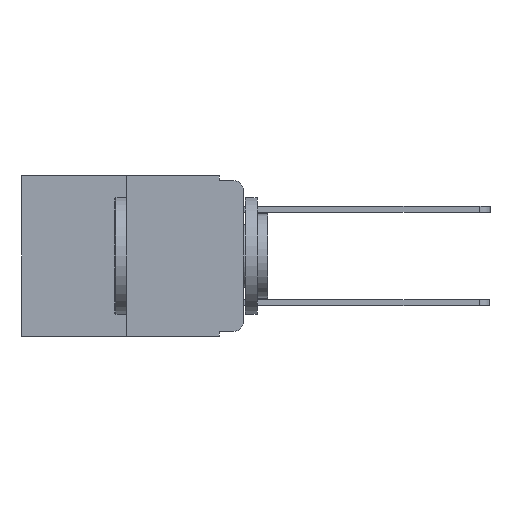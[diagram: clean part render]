
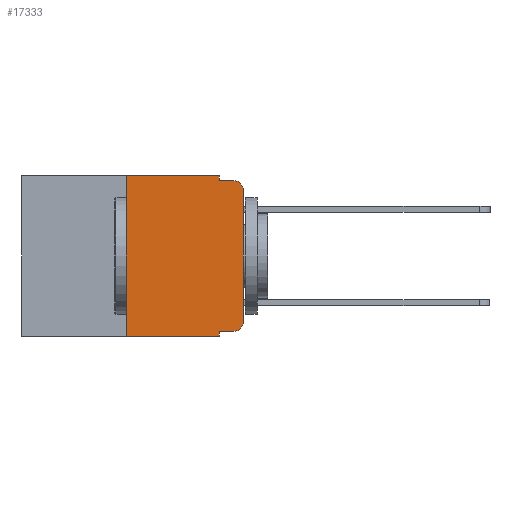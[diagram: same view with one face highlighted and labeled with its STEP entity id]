
A CAD part, left-side view. The second image highlights one B-rep face of the part: STEP entity #17333.
In plain terms, the highlighted planar face has unit normal (-1, 0, 0).
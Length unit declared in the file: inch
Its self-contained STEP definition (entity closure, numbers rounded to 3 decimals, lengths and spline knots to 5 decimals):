
#439 = CARTESIAN_POINT ( 'NONE',  ( 0., 0., -0.313 ) ) ;
#488 = CARTESIAN_POINT ( 'NONE',  ( 0., 0., 0. ) ) ;
#549 = VECTOR ( 'NONE', #4475, 39.37008 ) ;
#576 = CARTESIAN_POINT ( 'NONE',  ( 0., 0.473, 0. ) ) ;
#746 = DIRECTION ( 'NONE',  ( 0., 0., -1. ) ) ;
#815 = VERTEX_POINT ( 'NONE', #5910 ) ;
#910 = CARTESIAN_POINT ( 'NONE',  ( 0., 0.25, 0. ) ) ;
#1171 = LINE ( 'NONE', #17532, #549 ) ;
#1266 = VERTEX_POINT ( 'NONE', #5504 ) ;
#1741 = CIRCLE ( 'NONE', #10800, 0.02 ) ;
#1796 = VERTEX_POINT ( 'NONE', #20840 ) ;
#1843 = VERTEX_POINT ( 'NONE', #439 ) ;
#2025 = AXIS2_PLACEMENT_3D ( 'NONE', #576, #13933, #2569 ) ;
#2287 = CARTESIAN_POINT ( 'NONE',  ( 0., 0.051, -0.343 ) ) ;
#2481 = DIRECTION ( 'NONE',  ( 0., 0., 1. ) ) ;
#2569 = DIRECTION ( 'NONE',  ( 0., 0., -1. ) ) ;
#2634 = ORIENTED_EDGE ( 'NONE', *, *, #16061, .T. ) ;
#2987 = LINE ( 'NONE', #488, #16797 ) ;
#3080 = ORIENTED_EDGE ( 'NONE', *, *, #11273, .T. ) ;
#3301 = ORIENTED_EDGE ( 'NONE', *, *, #13153, .F. ) ;
#3503 = EDGE_CURVE ( 'NONE', #17056, #20672, #16402, .T. ) ;
#3620 = CARTESIAN_POINT ( 'NONE',  ( 0., 0.02, -0.01 ) ) ;
#3625 = ORIENTED_EDGE ( 'NONE', *, *, #6654, .T. ) ;
#3808 = ORIENTED_EDGE ( 'NONE', *, *, #7191, .F. ) ;
#3972 = EDGE_LOOP ( 'NONE', ( #4628, #7762, #17197, #21349, #4101, #3808, #3625, #3301, #3080, #2634 ) ) ;
#4101 = ORIENTED_EDGE ( 'NONE', *, *, #13943, .F. ) ;
#4105 = CARTESIAN_POINT ( 'NONE',  ( 0., 0.473, -0.343 ) ) ;
#4463 = VERTEX_POINT ( 'NONE', #2287 ) ;
#4475 = DIRECTION ( 'NONE',  ( 0., -1., 0. ) ) ;
#4520 = CARTESIAN_POINT ( 'NONE',  ( 0., 0.02, -0.313 ) ) ;
#4608 = LINE ( 'NONE', #11537, #22492 ) ;
#4628 = ORIENTED_EDGE ( 'NONE', *, *, #20937, .T. ) ;
#5504 = CARTESIAN_POINT ( 'NONE',  ( 0., 0.051, 0. ) ) ;
#5910 = CARTESIAN_POINT ( 'NONE',  ( 0., 0.25, -0.343 ) ) ;
#6438 = DIRECTION ( 'NONE',  ( 0., 0., -1. ) ) ;
#6467 = VECTOR ( 'NONE', #9586, 39.37008 ) ;
#6654 = EDGE_CURVE ( 'NONE', #815, #4463, #15599, .T. ) ;
#6898 = VERTEX_POINT ( 'NONE', #910 ) ;
#7191 = EDGE_CURVE ( 'NONE', #815, #6898, #23216, .T. ) ;
#7267 = CARTESIAN_POINT ( 'NONE',  ( 0., 0.02, -0.333 ) ) ;
#7762 = ORIENTED_EDGE ( 'NONE', *, *, #11163, .T. ) ;
#8779 = CARTESIAN_POINT ( 'NONE',  ( 0., 0.051, -0.333 ) ) ;
#8798 = CARTESIAN_POINT ( 'NONE',  ( 0., 0.051, 0. ) ) ;
#8963 = CIRCLE ( 'NONE', #15830, 0.02 ) ;
#9578 = LINE ( 'NONE', #8779, #13952 ) ;
#9586 = DIRECTION ( 'NONE',  ( 0., -1., 0. ) ) ;
#10800 = AXIS2_PLACEMENT_3D ( 'NONE', #23080, #12233, #746 ) ;
#11163 = EDGE_CURVE ( 'NONE', #1796, #20672, #1741, .T. ) ;
#11273 = EDGE_CURVE ( 'NONE', #15095, #22712, #9578, .T. ) ;
#11386 = CARTESIAN_POINT ( 'NONE',  ( 0., 0.25, 0. ) ) ;
#11537 = CARTESIAN_POINT ( 'NONE',  ( 0., 0.051, 0. ) ) ;
#12068 = PLANE ( 'NONE',  #2025 ) ;
#12233 = DIRECTION ( 'NONE',  ( -1., 0., 0. ) ) ;
#13153 = EDGE_CURVE ( 'NONE', #15095, #4463, #4608, .T. ) ;
#13527 = DIRECTION ( 'NONE',  ( 0., -1., 0. ) ) ;
#13933 = DIRECTION ( 'NONE',  ( 1., 0., 0. ) ) ;
#13943 = EDGE_CURVE ( 'NONE', #6898, #1266, #1171, .T. ) ;
#13952 = VECTOR ( 'NONE', #19811, 39.37008 ) ;
#14111 = EDGE_CURVE ( 'NONE', #1266, #17056, #21904, .T. ) ;
#14778 = CARTESIAN_POINT ( 'NONE',  ( 0., 0.051, -0.01 ) ) ;
#15026 = VECTOR ( 'NONE', #13527, 39.37008 ) ;
#15095 = VERTEX_POINT ( 'NONE', #22817 ) ;
#15599 = LINE ( 'NONE', #4105, #15026 ) ;
#15830 = AXIS2_PLACEMENT_3D ( 'NONE', #4520, #17580, #6438 ) ;
#16004 = VECTOR ( 'NONE', #23408, 39.37008 ) ;
#16061 = EDGE_CURVE ( 'NONE', #22712, #1843, #8963, .T. ) ;
#16402 = LINE ( 'NONE', #14778, #6467 ) ;
#16797 = VECTOR ( 'NONE', #2481, 39.37008 ) ;
#17056 = VERTEX_POINT ( 'NONE', #23959 ) ;
#17197 = ORIENTED_EDGE ( 'NONE', *, *, #3503, .F. ) ;
#17333 = ADVANCED_FACE ( 'NONE', ( #18134 ), #12068, .F. ) ;
#17532 = CARTESIAN_POINT ( 'NONE',  ( 0., 0.473, 0. ) ) ;
#17580 = DIRECTION ( 'NONE',  ( -1., 0., 0. ) ) ;
#18134 = FACE_OUTER_BOUND ( 'NONE', #3972, .T. ) ;
#19811 = DIRECTION ( 'NONE',  ( 0., -1., 0. ) ) ;
#20160 = VECTOR ( 'NONE', #24081, 39.37008 ) ;
#20625 = DIRECTION ( 'NONE',  ( 0., 0., -1. ) ) ;
#20672 = VERTEX_POINT ( 'NONE', #3620 ) ;
#20840 = CARTESIAN_POINT ( 'NONE',  ( 0., 0., -0.03 ) ) ;
#20937 = EDGE_CURVE ( 'NONE', #1843, #1796, #2987, .T. ) ;
#21349 = ORIENTED_EDGE ( 'NONE', *, *, #14111, .F. ) ;
#21904 = LINE ( 'NONE', #8798, #16004 ) ;
#22492 = VECTOR ( 'NONE', #20625, 39.37008 ) ;
#22712 = VERTEX_POINT ( 'NONE', #7267 ) ;
#22817 = CARTESIAN_POINT ( 'NONE',  ( 0., 0.051, -0.333 ) ) ;
#23080 = CARTESIAN_POINT ( 'NONE',  ( 0., 0.02, -0.03 ) ) ;
#23216 = LINE ( 'NONE', #11386, #20160 ) ;
#23408 = DIRECTION ( 'NONE',  ( 0., 0., -1. ) ) ;
#23959 = CARTESIAN_POINT ( 'NONE',  ( 0., 0.051, -0.01 ) ) ;
#24081 = DIRECTION ( 'NONE',  ( 0., 0., 1. ) ) ;
